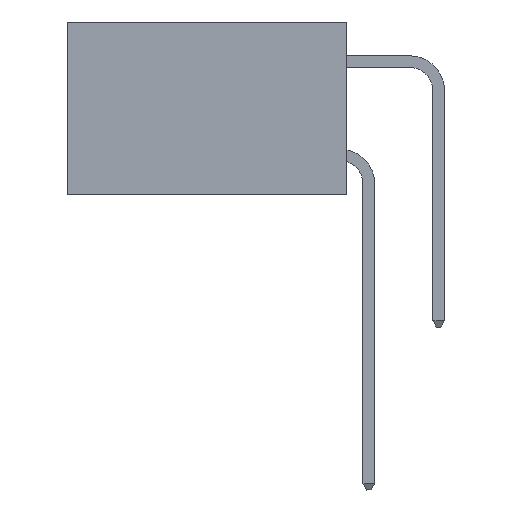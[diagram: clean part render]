
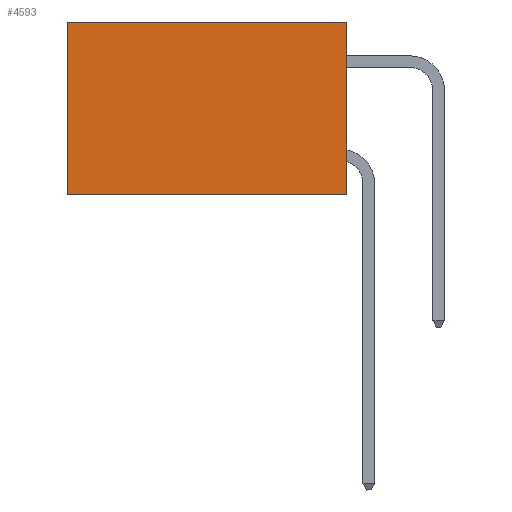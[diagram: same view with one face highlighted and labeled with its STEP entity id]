
A CAD part, left-side view. The second image highlights one B-rep face of the part: STEP entity #4593.
In plain terms, the highlighted planar face has unit normal (-1, 0, 0).
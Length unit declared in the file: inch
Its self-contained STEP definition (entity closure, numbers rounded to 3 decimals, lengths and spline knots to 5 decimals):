
#316 = ORIENTED_EDGE ( 'NONE', *, *, #8609, .F. ) ;
#663 = VERTEX_POINT ( 'NONE', #10502 ) ;
#852 = LINE ( 'NONE', #16498, #12985 ) ;
#1257 = DIRECTION ( 'NONE',  ( 1., 0., 0. ) ) ;
#1345 = LINE ( 'NONE', #4267, #14067 ) ;
#1827 = CARTESIAN_POINT ( 'NONE',  ( 0.2875, 0., -0.37 ) ) ;
#2094 = LINE ( 'NONE', #16473, #14420 ) ;
#2514 = EDGE_CURVE ( 'NONE', #10436, #14291, #2094, .T. ) ;
#3149 = DIRECTION ( 'NONE',  ( 0., 0., -1. ) ) ;
#4094 = EDGE_CURVE ( 'NONE', #663, #10387, #10273, .T. ) ;
#4267 = CARTESIAN_POINT ( 'NONE',  ( 0.2875, 0., 0. ) ) ;
#4412 = CARTESIAN_POINT ( 'NONE',  ( 0.2875, 0.6, 0. ) ) ;
#4593 = ADVANCED_FACE ( 'NONE', ( #5059 ), #9101, .F. ) ;
#5059 = FACE_OUTER_BOUND ( 'NONE', #16703, .T. ) ;
#6455 = VECTOR ( 'NONE', #3149, 39.37008 ) ;
#6568 = ORIENTED_EDGE ( 'NONE', *, *, #6751, .T. ) ;
#6751 = EDGE_CURVE ( 'NONE', #10436, #663, #1345, .T. ) ;
#6894 = DIRECTION ( 'NONE',  ( 0., 1., 0. ) ) ;
#7751 = CARTESIAN_POINT ( 'NONE',  ( 0.2875, 0., 0. ) ) ;
#8609 = EDGE_CURVE ( 'NONE', #14291, #10387, #852, .T. ) ;
#8732 = DIRECTION ( 'NONE',  ( 0., 1., 0. ) ) ;
#9101 = PLANE ( 'NONE',  #15657 ) ;
#10273 = LINE ( 'NONE', #4412, #6455 ) ;
#10387 = VERTEX_POINT ( 'NONE', #16180 ) ;
#10436 = VERTEX_POINT ( 'NONE', #16342 ) ;
#10502 = CARTESIAN_POINT ( 'NONE',  ( 0.2875, 0.6, 0. ) ) ;
#12015 = ORIENTED_EDGE ( 'NONE', *, *, #2514, .F. ) ;
#12985 = VECTOR ( 'NONE', #8732, 39.37008 ) ;
#13416 = ORIENTED_EDGE ( 'NONE', *, *, #4094, .T. ) ;
#14067 = VECTOR ( 'NONE', #6894, 39.37008 ) ;
#14291 = VERTEX_POINT ( 'NONE', #1827 ) ;
#14420 = VECTOR ( 'NONE', #16313, 39.37008 ) ;
#15657 = AXIS2_PLACEMENT_3D ( 'NONE', #7751, #1257, #16133 ) ;
#16133 = DIRECTION ( 'NONE',  ( 0., 0., -1. ) ) ;
#16180 = CARTESIAN_POINT ( 'NONE',  ( 0.2875, 0.6, -0.37 ) ) ;
#16313 = DIRECTION ( 'NONE',  ( 0., 0., -1. ) ) ;
#16342 = CARTESIAN_POINT ( 'NONE',  ( 0.2875, 0., 0. ) ) ;
#16473 = CARTESIAN_POINT ( 'NONE',  ( 0.2875, 0., 0. ) ) ;
#16498 = CARTESIAN_POINT ( 'NONE',  ( 0.2875, 0., -0.37 ) ) ;
#16703 = EDGE_LOOP ( 'NONE', ( #13416, #316, #12015, #6568 ) ) ;
